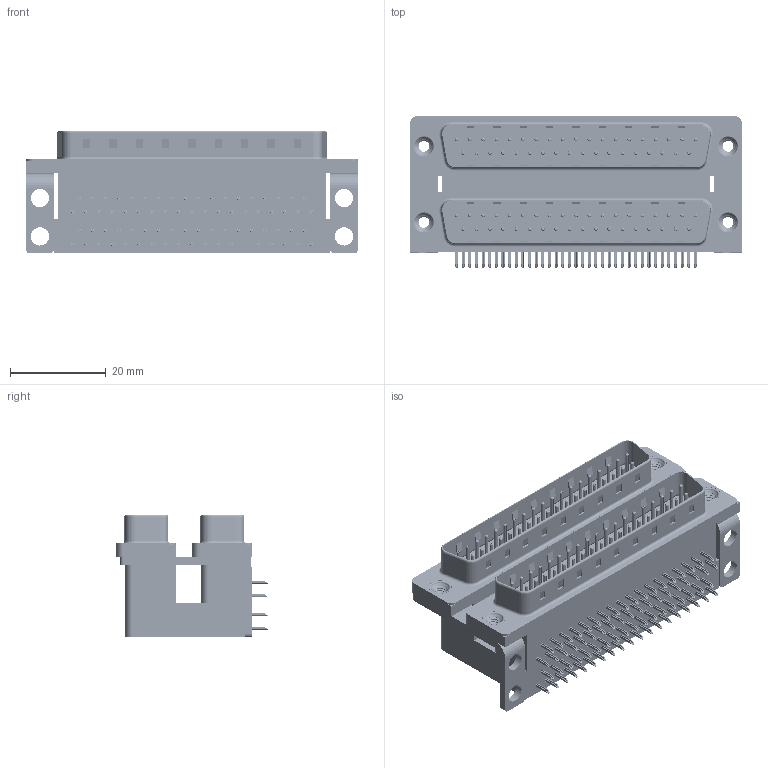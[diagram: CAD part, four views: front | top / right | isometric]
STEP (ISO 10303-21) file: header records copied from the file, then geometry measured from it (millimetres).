
FILE_DESCRIPTION (( 'STEP AP203' ), '1' );
FILE_NAME ('661-037-664-002.STEP', '2022-06-14T20:48:52', ( '' ), ( '' ), 'SwSTEP 2.0', 'SolidWorks 2020', '' );
FILE_SCHEMA (( 'CONFIG_CONTROL_DESIGN' ));
Length unit declared in the file: millimetre
Products named in the file (11): 661 Housing Upper_37 Contacts L; 661 Threaded Rivet_4-40; 661 Contact Top Upper_L; 661 Contact Bottom Upper_L; 661-037-664-002; 661 Housing Spacer_37 Contacts L; 661 Mounting Bracket_NoneL; 661 Shell_37 Contacts; 661 Contact Bottom Lower; 661 Housing Lower_37 Contacts; 661 Contact Top Lower
Assembly tree (85 placements, depth 2):
  661-037-664-002
    661 Housing Lower_37 Contacts
    661 Housing Spacer_37 Contacts L
    661 Housing Upper_37 Contacts L
    661 Shell_37 Contacts  x2
    661 Contact Bottom Lower  x18
    661 Contact Top Lower  x19
    661 Contact Bottom Upper_L  x18
    661 Contact Top Upper_L  x19
    661 Mounting Bracket_NoneL  x2
    661 Threaded Rivet_4-40  x4
Bounding box: 69.32 x 31.61 x 25.6 mm (x, y, z)
Volume: 27918.5 mm3; surface area: 28515.6 mm2
Topology: 85 solids, 85 shells, 6582 faces, 16332 edges, 10094 vertices
Faces by surface type: plane 4250, cylinder 1794, torus 506, cone 20, bspline 12
Entity records: 50706 total; most frequent: CARTESIAN_POINT 9774, DIRECTION 7745, ORIENTED_EDGE 7640, EDGE_CURVE 3820, VECTOR 3003, LINE 3003, VERTEX_POINT 2482, AXIS2_PLACEMENT_3D 2371
